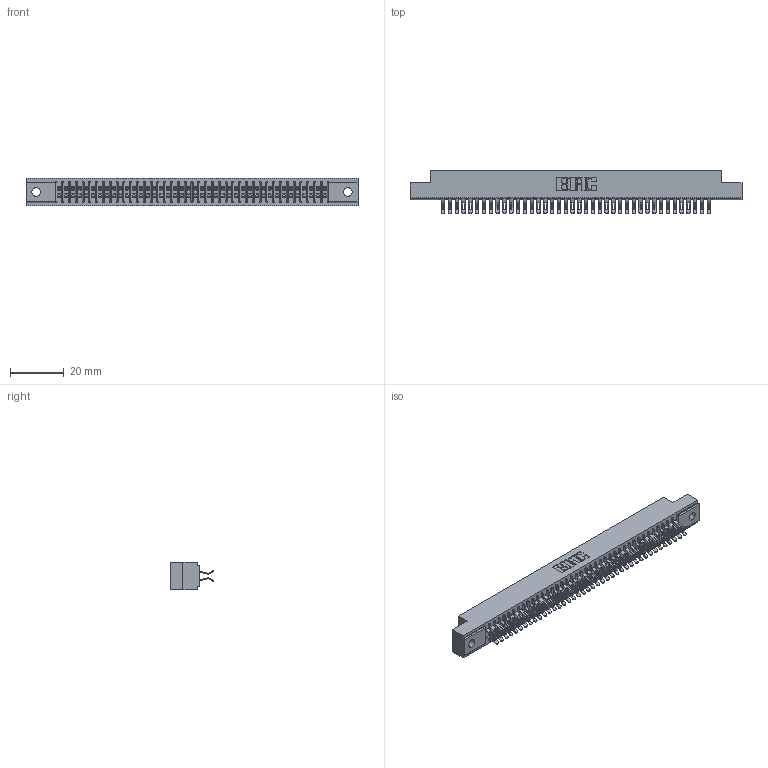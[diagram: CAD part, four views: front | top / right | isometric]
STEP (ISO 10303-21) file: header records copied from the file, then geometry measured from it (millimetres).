
FILE_DESCRIPTION (( 'STEP AP203' ), '1' );
FILE_NAME ('391-080-555-202.STEP', '2018-08-09T15:43:37', ( '' ), ( '' ), 'SwSTEP 2.0', 'SolidWorks 2016', '' );
FILE_SCHEMA (( 'CONFIG_CONTROL_DESIGN' ));
Length unit declared in the file: inch
Products named in the file (3): 341 Part_.128 (3.25) Dia Mounting Holes; 341-292-001_341-292-155; 391-080-555-202
Assembly tree (81 placements, depth 2):
  391-080-555-202
    341 Part_.128 (3.25) Dia Mounting Holes
    341-292-001_341-292-155  x80
Bounding box: 123.83 x 16.31 x 10.16 mm (x, y, z)
Volume: 9203.6 mm3; surface area: 16676.5 mm2
Topology: 81 solids, 81 shells, 6356 faces, 18996 edges, 12366 vertices
Faces by surface type: plane 3428, cylinder 2768, sphere 82, torus 78
Entity records: 49147 total; most frequent: CARTESIAN_POINT 8186, ORIENTED_EDGE 8124, DIRECTION 7936, EDGE_CURVE 4062, LINE 3264, VECTOR 3264, VERTEX_POINT 2570, AXIS2_PLACEMENT_3D 2336
